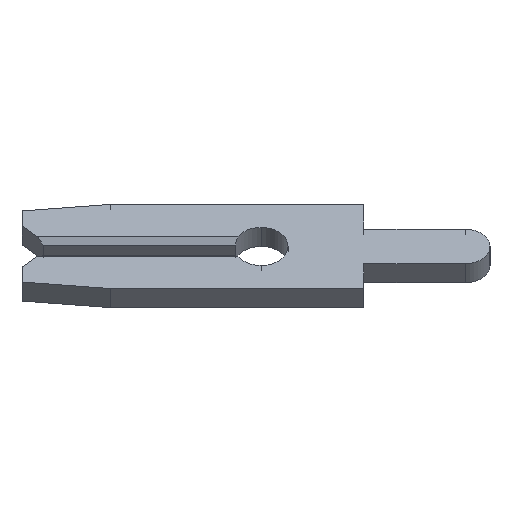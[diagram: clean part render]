
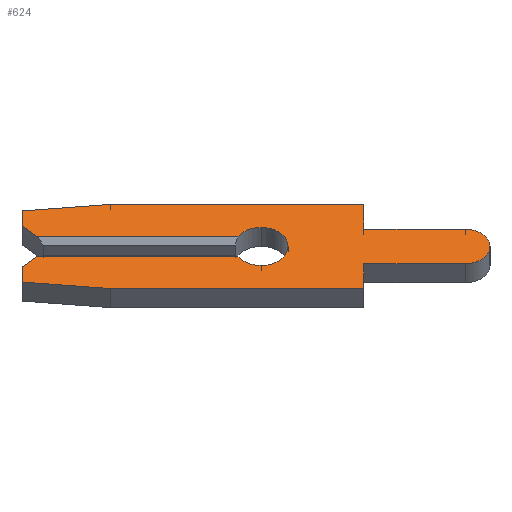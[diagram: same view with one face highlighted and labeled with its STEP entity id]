
A CAD part, left-side view. The second image highlights one B-rep face of the part: STEP entity #624.
In plain terms, the highlighted face is planar.
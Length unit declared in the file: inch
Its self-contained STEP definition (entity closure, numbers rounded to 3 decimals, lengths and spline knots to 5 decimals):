
#4 = CARTESIAN_POINT ( 'NONE',  ( -0.013, -0.099, 0.0575 ) ) ;
#13 = VECTOR ( 'NONE', #955, 39.37008 ) ;
#17 = VECTOR ( 'NONE', #1160, 39.37008 ) ;
#21 = EDGE_CURVE ( 'NONE', #430, #1036, #784, .T. ) ;
#23 = EDGE_CURVE ( 'NONE', #614, #995, #98, .T. ) ;
#30 = LINE ( 'NONE', #435, #81 ) ;
#65 = EDGE_CURVE ( 'NONE', #813, #195, #338, .T. ) ;
#71 = EDGE_CURVE ( 'NONE', #965, #531, #306, .T. ) ;
#72 = CARTESIAN_POINT ( 'NONE',  ( -0.013, 0.216, 0.013 ) ) ;
#76 = DIRECTION ( 'NONE',  ( 0., 0., -1. ) ) ;
#78 = ORIENTED_EDGE ( 'NONE', *, *, #725, .F. ) ;
#81 = VECTOR ( 'NONE', #1041, 39.37008 ) ;
#92 = EDGE_LOOP ( 'NONE', ( #1086, #984, #252, #78, #1380, #991, #451, #542, #299, #219, #591, #886, #487, #1290, #361, #452, #1042, #1341 ) ) ;
#94 = VERTEX_POINT ( 'NONE', #1138 ) ;
#97 = CARTESIAN_POINT ( 'NONE',  ( -0.013, -0.099, 0.0235 ) ) ;
#98 = CIRCLE ( 'NONE', #720, 0.026 ) ;
#121 = CARTESIAN_POINT ( 'NONE',  ( -0.013, 0.146, -0.0575 ) ) ;
#127 = LINE ( 'NONE', #272, #864 ) ;
#157 = DIRECTION ( 'NONE',  ( 1., 0., 0. ) ) ;
#158 = EDGE_CURVE ( 'NONE', #868, #831, #1331, .T. ) ;
#171 = DIRECTION ( 'NONE',  ( 0., 0., -1. ) ) ;
#189 = LINE ( 'NONE', #1304, #1046 ) ;
#191 = CIRCLE ( 'NONE', #456, 0.0235 ) ;
#195 = VERTEX_POINT ( 'NONE', #1165 ) ;
#219 = ORIENTED_EDGE ( 'NONE', *, *, #21, .F. ) ;
#234 = EDGE_CURVE ( 'NONE', #1245, #430, #968, .T. ) ;
#235 = AXIS2_PLACEMENT_3D ( 'NONE', #1255, #1130, #171 ) ;
#247 = DIRECTION ( 'NONE',  ( 0., 0., -1. ) ) ;
#250 = VECTOR ( 'NONE', #1088, 39.37008 ) ;
#252 = ORIENTED_EDGE ( 'NONE', *, *, #23, .F. ) ;
#253 = CARTESIAN_POINT ( 'NONE',  ( -0.013, 0., 0. ) ) ;
#272 = CARTESIAN_POINT ( 'NONE',  ( -0.013, 0.231, 0.04857 ) ) ;
#276 = CARTESIAN_POINT ( 'NONE',  ( -0.013, 0.146, 0.0575 ) ) ;
#280 = LINE ( 'NONE', #4, #557 ) ;
#281 = DIRECTION ( 'NONE',  ( 1., 0., 0. ) ) ;
#285 = EDGE_CURVE ( 'NONE', #1036, #635, #1383, .T. ) ;
#293 = CARTESIAN_POINT ( 'NONE',  ( -0.013, 0., -0.026 ) ) ;
#299 = ORIENTED_EDGE ( 'NONE', *, *, #285, .F. ) ;
#306 = LINE ( 'NONE', #836, #17 ) ;
#324 = VECTOR ( 'NONE', #633, 39.37008 ) ;
#338 = LINE ( 'NONE', #1050, #1153 ) ;
#361 = ORIENTED_EDGE ( 'NONE', *, *, #158, .F. ) ;
#368 = CARTESIAN_POINT ( 'NONE',  ( -0.013, 0.231, -0.04857 ) ) ;
#378 = CARTESIAN_POINT ( 'NONE',  ( -0.013, -0.1975, 0. ) ) ;
#395 = EDGE_CURVE ( 'NONE', #94, #1245, #191, .T. ) ;
#397 = DIRECTION ( 'NONE',  ( 0., 0., -1. ) ) ;
#407 = VERTEX_POINT ( 'NONE', #1323 ) ;
#420 = CARTESIAN_POINT ( 'NONE',  ( -0.013, 0., 0.026 ) ) ;
#430 = VERTEX_POINT ( 'NONE', #1011 ) ;
#435 = CARTESIAN_POINT ( 'NONE',  ( -0.013, 0.2105, 0.0075 ) ) ;
#451 = ORIENTED_EDGE ( 'NONE', *, *, #1370, .F. ) ;
#452 = ORIENTED_EDGE ( 'NONE', *, *, #748, .F. ) ;
#456 = AXIS2_PLACEMENT_3D ( 'NONE', #378, #157, #489 ) ;
#465 = EDGE_CURVE ( 'NONE', #995, #1272, #1345, .T. ) ;
#487 = ORIENTED_EDGE ( 'NONE', *, *, #1047, .F. ) ;
#489 = DIRECTION ( 'NONE',  ( 0., 0., 1. ) ) ;
#506 = EDGE_CURVE ( 'NONE', #635, #407, #1186, .T. ) ;
#531 = VERTEX_POINT ( 'NONE', #1221 ) ;
#542 = ORIENTED_EDGE ( 'NONE', *, *, #506, .F. ) ;
#557 = VECTOR ( 'NONE', #1062, 39.37008 ) ;
#578 = CARTESIAN_POINT ( 'NONE',  ( -0.013, 0.146, -0.0575 ) ) ;
#580 = CARTESIAN_POINT ( 'NONE',  ( -0.013, 0.231, -0.028 ) ) ;
#581 = CARTESIAN_POINT ( 'NONE',  ( -0.013, 0., 0. ) ) ;
#591 = ORIENTED_EDGE ( 'NONE', *, *, #234, .F. ) ;
#604 = CARTESIAN_POINT ( 'NONE',  ( -0.013, -0.099, 0.0235 ) ) ;
#613 = CARTESIAN_POINT ( 'NONE',  ( -0.013, 0., 0. ) ) ;
#614 = VERTEX_POINT ( 'NONE', #293 ) ;
#619 = LINE ( 'NONE', #97, #13 ) ;
#624 = ADVANCED_FACE ( 'NONE', ( #1294 ), #1142, .F. ) ;
#633 = DIRECTION ( 'NONE',  ( 0., -0.707, 0.707 ) ) ;
#635 = VERTEX_POINT ( 'NONE', #578 ) ;
#645 = DIRECTION ( 'NONE',  ( 0., -1., 0. ) ) ;
#656 = DIRECTION ( 'NONE',  ( 0., 1., 0. ) ) ;
#666 = VERTEX_POINT ( 'NONE', #1135 ) ;
#671 = AXIS2_PLACEMENT_3D ( 'NONE', #613, #281, #397 ) ;
#675 = VECTOR ( 'NONE', #76, 39.37008 ) ;
#720 = AXIS2_PLACEMENT_3D ( 'NONE', #253, #1100, #247 ) ;
#725 = EDGE_CURVE ( 'NONE', #195, #614, #896, .T. ) ;
#731 = VERTEX_POINT ( 'NONE', #604 ) ;
#738 = VECTOR ( 'NONE', #656, 39.37008 ) ;
#748 = EDGE_CURVE ( 'NONE', #531, #868, #127, .T. ) ;
#784 = LINE ( 'NONE', #945, #675 ) ;
#804 = DIRECTION ( 'NONE',  ( 0., 0., -1. ) ) ;
#813 = VERTEX_POINT ( 'NONE', #1241 ) ;
#829 = DIRECTION ( 'NONE',  ( 0., -1., 0. ) ) ;
#831 = VERTEX_POINT ( 'NONE', #1126 ) ;
#836 = CARTESIAN_POINT ( 'NONE',  ( -0.013, 0.231, 0.028 ) ) ;
#864 = VECTOR ( 'NONE', #1019, 39.37008 ) ;
#865 = VECTOR ( 'NONE', #875, 39.37008 ) ;
#868 = VERTEX_POINT ( 'NONE', #276 ) ;
#875 = DIRECTION ( 'NONE',  ( 0., 0., 1. ) ) ;
#878 = AXIS2_PLACEMENT_3D ( 'NONE', #581, #1104, #804 ) ;
#881 = LINE ( 'NONE', #1265, #324 ) ;
#886 = ORIENTED_EDGE ( 'NONE', *, *, #395, .F. ) ;
#895 = VERTEX_POINT ( 'NONE', #72 ) ;
#896 = CIRCLE ( 'NONE', #235, 0.026 ) ;
#920 = LINE ( 'NONE', #580, #865 ) ;
#945 = CARTESIAN_POINT ( 'NONE',  ( -0.013, -0.099, -0.0575 ) ) ;
#955 = DIRECTION ( 'NONE',  ( 0., -1., 0. ) ) ;
#965 = VERTEX_POINT ( 'NONE', #1282 ) ;
#967 = CARTESIAN_POINT ( 'NONE',  ( -0.013, 0.02252, 0.013 ) ) ;
#968 = LINE ( 'NONE', #1094, #250 ) ;
#984 = ORIENTED_EDGE ( 'NONE', *, *, #465, .F. ) ;
#991 = ORIENTED_EDGE ( 'NONE', *, *, #1026, .F. ) ;
#995 = VERTEX_POINT ( 'NONE', #420 ) ;
#1011 = CARTESIAN_POINT ( 'NONE',  ( -0.013, -0.099, -0.0235 ) ) ;
#1018 = VECTOR ( 'NONE', #645, 39.37008 ) ;
#1019 = DIRECTION ( 'NONE',  ( 0., -0.995, 0.105 ) ) ;
#1026 = EDGE_CURVE ( 'NONE', #666, #813, #881, .T. ) ;
#1036 = VERTEX_POINT ( 'NONE', #1163 ) ;
#1041 = DIRECTION ( 'NONE',  ( 0., 0.707, 0.707 ) ) ;
#1042 = ORIENTED_EDGE ( 'NONE', *, *, #71, .F. ) ;
#1046 = VECTOR ( 'NONE', #1184, 39.37008 ) ;
#1047 = EDGE_CURVE ( 'NONE', #731, #94, #619, .T. ) ;
#1050 = CARTESIAN_POINT ( 'NONE',  ( -0.013, 0., -0.013 ) ) ;
#1062 = DIRECTION ( 'NONE',  ( 0., 0., -1. ) ) ;
#1081 = CARTESIAN_POINT ( 'NONE',  ( -0.013, -0.1975, -0.0235 ) ) ;
#1086 = ORIENTED_EDGE ( 'NONE', *, *, #1305, .T. ) ;
#1088 = DIRECTION ( 'NONE',  ( 0., 1., 0. ) ) ;
#1094 = CARTESIAN_POINT ( 'NONE',  ( -0.013, -0.099, -0.0235 ) ) ;
#1100 = DIRECTION ( 'NONE',  ( -1., 0., 0. ) ) ;
#1104 = DIRECTION ( 'NONE',  ( -1., 0., 0. ) ) ;
#1121 = EDGE_CURVE ( 'NONE', #895, #965, #30, .T. ) ;
#1126 = CARTESIAN_POINT ( 'NONE',  ( -0.013, -0.099, 0.0575 ) ) ;
#1130 = DIRECTION ( 'NONE',  ( -1., 0., 0. ) ) ;
#1135 = CARTESIAN_POINT ( 'NONE',  ( -0.013, 0.231, -0.028 ) ) ;
#1138 = CARTESIAN_POINT ( 'NONE',  ( -0.013, -0.1975, 0.0235 ) ) ;
#1142 = PLANE ( 'NONE',  #671 ) ;
#1153 = VECTOR ( 'NONE', #829, 39.37008 ) ;
#1160 = DIRECTION ( 'NONE',  ( 0., 0., 1. ) ) ;
#1163 = CARTESIAN_POINT ( 'NONE',  ( -0.013, -0.099, -0.0575 ) ) ;
#1165 = CARTESIAN_POINT ( 'NONE',  ( -0.013, 0.02252, -0.013 ) ) ;
#1184 = DIRECTION ( 'NONE',  ( 0., -1., 0. ) ) ;
#1186 = LINE ( 'NONE', #368, #1223 ) ;
#1195 = EDGE_CURVE ( 'NONE', #831, #731, #280, .T. ) ;
#1221 = CARTESIAN_POINT ( 'NONE',  ( -0.013, 0.231, 0.04857 ) ) ;
#1223 = VECTOR ( 'NONE', #1233, 39.37008 ) ;
#1233 = DIRECTION ( 'NONE',  ( 0., 0.995, 0.105 ) ) ;
#1241 = CARTESIAN_POINT ( 'NONE',  ( -0.013, 0.216, -0.013 ) ) ;
#1245 = VERTEX_POINT ( 'NONE', #1081 ) ;
#1255 = CARTESIAN_POINT ( 'NONE',  ( -0.013, 0., 0. ) ) ;
#1265 = CARTESIAN_POINT ( 'NONE',  ( -0.013, 0.2105, -0.0075 ) ) ;
#1272 = VERTEX_POINT ( 'NONE', #967 ) ;
#1282 = CARTESIAN_POINT ( 'NONE',  ( -0.013, 0.231, 0.028 ) ) ;
#1290 = ORIENTED_EDGE ( 'NONE', *, *, #1195, .F. ) ;
#1294 = FACE_OUTER_BOUND ( 'NONE', #92, .T. ) ;
#1300 = CARTESIAN_POINT ( 'NONE',  ( -0.013, 0.146, 0.0575 ) ) ;
#1304 = CARTESIAN_POINT ( 'NONE',  ( -0.013, 0.231, 0.013 ) ) ;
#1305 = EDGE_CURVE ( 'NONE', #895, #1272, #189, .T. ) ;
#1323 = CARTESIAN_POINT ( 'NONE',  ( -0.013, 0.231, -0.04857 ) ) ;
#1331 = LINE ( 'NONE', #1300, #1018 ) ;
#1341 = ORIENTED_EDGE ( 'NONE', *, *, #1121, .F. ) ;
#1345 = CIRCLE ( 'NONE', #878, 0.026 ) ;
#1370 = EDGE_CURVE ( 'NONE', #407, #666, #920, .T. ) ;
#1380 = ORIENTED_EDGE ( 'NONE', *, *, #65, .F. ) ;
#1383 = LINE ( 'NONE', #121, #738 ) ;
